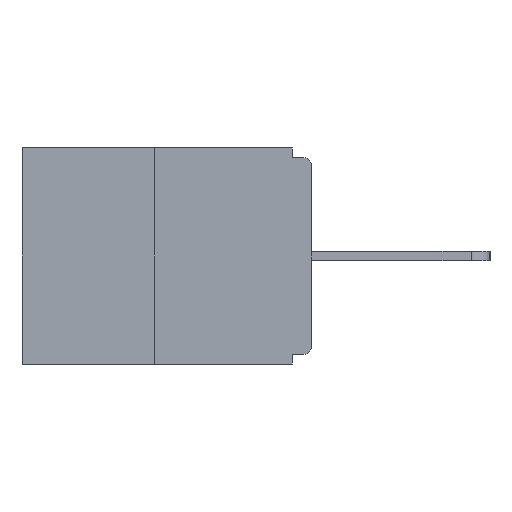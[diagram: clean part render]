
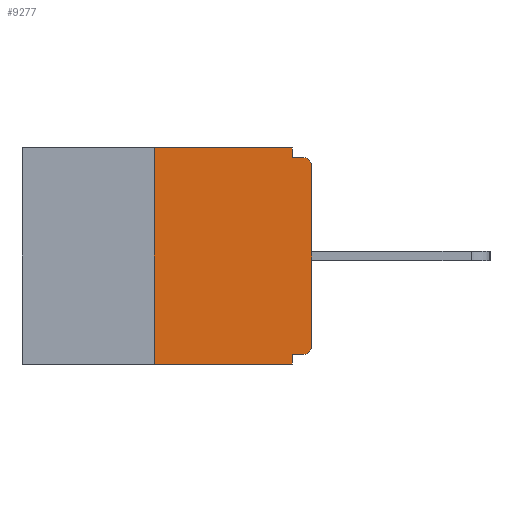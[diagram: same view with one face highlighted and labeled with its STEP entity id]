
A CAD part, left-side view. The second image highlights one B-rep face of the part: STEP entity #9277.
In plain terms, the highlighted planar face has unit normal (-1, 0, 0).
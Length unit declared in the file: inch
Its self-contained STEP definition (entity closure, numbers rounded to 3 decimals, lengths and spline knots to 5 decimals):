
#47 = CARTESIAN_POINT ( 'NONE',  ( 0., 0., -0.015 ) ) ;
#317 = DIRECTION ( 'NONE',  ( 0., 1., 0. ) ) ;
#396 = CARTESIAN_POINT ( 'NONE',  ( 0., 0.25, 0. ) ) ;
#550 = CIRCLE ( 'NONE', #8208, 0.015 ) ;
#909 = VERTEX_POINT ( 'NONE', #8559 ) ;
#1046 = DIRECTION ( 'NONE',  ( 0., 0., 1. ) ) ;
#1180 = VECTOR ( 'NONE', #14859, 39.37008 ) ;
#1407 = LINE ( 'NONE', #47, #1180 ) ;
#1647 = VECTOR ( 'NONE', #11227, 39.37008 ) ;
#1730 = CARTESIAN_POINT ( 'NONE',  ( 0., 0., -0.328 ) ) ;
#1750 = VECTOR ( 'NONE', #12781, 39.37008 ) ;
#1773 = DIRECTION ( 'NONE',  ( -1., 0., 0. ) ) ;
#2042 = EDGE_CURVE ( 'NONE', #14101, #11144, #2411, .T. ) ;
#2411 = LINE ( 'NONE', #2553, #12735 ) ;
#2553 = CARTESIAN_POINT ( 'NONE',  ( 0., 0., 0. ) ) ;
#2626 = ORIENTED_EDGE ( 'NONE', *, *, #10121, .F. ) ;
#2649 = CARTESIAN_POINT ( 'NONE',  ( 0., 0., -0.313 ) ) ;
#3064 = ORIENTED_EDGE ( 'NONE', *, *, #10946, .T. ) ;
#3123 = EDGE_LOOP ( 'NONE', ( #6985, #7214, #9758, #12051, #2626, #3064, #4207, #6616, #13733, #9381 ) ) ;
#3523 = DIRECTION ( 'NONE',  ( 0., 0., -1. ) ) ;
#3637 = LINE ( 'NONE', #9335, #1750 ) ;
#3724 = VECTOR ( 'NONE', #7939, 39.37008 ) ;
#3832 = CARTESIAN_POINT ( 'NONE',  ( 0., 0.25, -0.343 ) ) ;
#4206 = VERTEX_POINT ( 'NONE', #8380 ) ;
#4207 = ORIENTED_EDGE ( 'NONE', *, *, #2042, .T. ) ;
#4418 = VERTEX_POINT ( 'NONE', #11089 ) ;
#4456 = EDGE_CURVE ( 'NONE', #4206, #909, #5824, .T. ) ;
#5024 = VERTEX_POINT ( 'NONE', #8567 ) ;
#5153 = EDGE_CURVE ( 'NONE', #5024, #6578, #14577, .T. ) ;
#5521 = CARTESIAN_POINT ( 'NONE',  ( 0., 0., -0.03 ) ) ;
#5589 = DIRECTION ( 'NONE',  ( 0., 0., -1. ) ) ;
#5775 = FACE_OUTER_BOUND ( 'NONE', #3123, .T. ) ;
#5824 = LINE ( 'NONE', #10176, #3724 ) ;
#5860 = DIRECTION ( 'NONE',  ( 0., 0., 1. ) ) ;
#5984 = AXIS2_PLACEMENT_3D ( 'NONE', #9222, #13804, #3523 ) ;
#6578 = VERTEX_POINT ( 'NONE', #9167 ) ;
#6616 = ORIENTED_EDGE ( 'NONE', *, *, #7360, .T. ) ;
#6860 = AXIS2_PLACEMENT_3D ( 'NONE', #9583, #1773, #10788 ) ;
#6985 = ORIENTED_EDGE ( 'NONE', *, *, #7396, .F. ) ;
#7214 = ORIENTED_EDGE ( 'NONE', *, *, #12760, .F. ) ;
#7360 = EDGE_CURVE ( 'NONE', #11144, #4418, #550, .T. ) ;
#7396 = EDGE_CURVE ( 'NONE', #8554, #4206, #3637, .T. ) ;
#7939 = DIRECTION ( 'NONE',  ( 0., 0., -1. ) ) ;
#7997 = CARTESIAN_POINT ( 'NONE',  ( 0., 0.015, -0.03 ) ) ;
#8208 = AXIS2_PLACEMENT_3D ( 'NONE', #7997, #11525, #5589 ) ;
#8380 = CARTESIAN_POINT ( 'NONE',  ( 0., 0.031, 0. ) ) ;
#8554 = VERTEX_POINT ( 'NONE', #396 ) ;
#8559 = CARTESIAN_POINT ( 'NONE',  ( 0., 0.031, -0.015 ) ) ;
#8567 = CARTESIAN_POINT ( 'NONE',  ( 0., 0.031, -0.328 ) ) ;
#8672 = LINE ( 'NONE', #10094, #1647 ) ;
#9078 = CARTESIAN_POINT ( 'NONE',  ( 0., 0.25, 0. ) ) ;
#9167 = CARTESIAN_POINT ( 'NONE',  ( 0., 0.031, -0.343 ) ) ;
#9222 = CARTESIAN_POINT ( 'NONE',  ( 0., 0.46, 0. ) ) ;
#9254 = EDGE_CURVE ( 'NONE', #909, #4418, #1407, .T. ) ;
#9277 = ADVANCED_FACE ( 'NONE', ( #5775 ), #10344, .F. ) ;
#9335 = CARTESIAN_POINT ( 'NONE',  ( 0., 0.46, 0. ) ) ;
#9381 = ORIENTED_EDGE ( 'NONE', *, *, #4456, .F. ) ;
#9583 = CARTESIAN_POINT ( 'NONE',  ( 0., 0.015, -0.313 ) ) ;
#9758 = ORIENTED_EDGE ( 'NONE', *, *, #11175, .T. ) ;
#10094 = CARTESIAN_POINT ( 'NONE',  ( 0., 0.46, -0.343 ) ) ;
#10121 = EDGE_CURVE ( 'NONE', #14429, #5024, #11041, .T. ) ;
#10176 = CARTESIAN_POINT ( 'NONE',  ( 0., 0.031, 0. ) ) ;
#10344 = PLANE ( 'NONE',  #5984 ) ;
#10509 = VERTEX_POINT ( 'NONE', #3832 ) ;
#10788 = DIRECTION ( 'NONE',  ( 0., 0., -1. ) ) ;
#10946 = EDGE_CURVE ( 'NONE', #14429, #14101, #13099, .T. ) ;
#11041 = LINE ( 'NONE', #1730, #12155 ) ;
#11079 = VECTOR ( 'NONE', #12160, 39.37008 ) ;
#11089 = CARTESIAN_POINT ( 'NONE',  ( 0., 0.015, -0.015 ) ) ;
#11113 = CARTESIAN_POINT ( 'NONE',  ( 0., 0.031, -0.343 ) ) ;
#11144 = VERTEX_POINT ( 'NONE', #5521 ) ;
#11175 = EDGE_CURVE ( 'NONE', #10509, #6578, #8672, .T. ) ;
#11227 = DIRECTION ( 'NONE',  ( 0., -1., 0. ) ) ;
#11338 = LINE ( 'NONE', #9078, #11749 ) ;
#11525 = DIRECTION ( 'NONE',  ( -1., 0., 0. ) ) ;
#11749 = VECTOR ( 'NONE', #1046, 39.37008 ) ;
#12051 = ORIENTED_EDGE ( 'NONE', *, *, #5153, .F. ) ;
#12155 = VECTOR ( 'NONE', #317, 39.37008 ) ;
#12160 = DIRECTION ( 'NONE',  ( 0., 0., -1. ) ) ;
#12735 = VECTOR ( 'NONE', #5860, 39.37008 ) ;
#12760 = EDGE_CURVE ( 'NONE', #10509, #8554, #11338, .T. ) ;
#12781 = DIRECTION ( 'NONE',  ( 0., -1., 0. ) ) ;
#13099 = CIRCLE ( 'NONE', #6860, 0.015 ) ;
#13733 = ORIENTED_EDGE ( 'NONE', *, *, #9254, .F. ) ;
#13804 = DIRECTION ( 'NONE',  ( 1., 0., 0. ) ) ;
#13944 = CARTESIAN_POINT ( 'NONE',  ( 0., 0.015, -0.328 ) ) ;
#14101 = VERTEX_POINT ( 'NONE', #2649 ) ;
#14429 = VERTEX_POINT ( 'NONE', #13944 ) ;
#14577 = LINE ( 'NONE', #11113, #11079 ) ;
#14859 = DIRECTION ( 'NONE',  ( 0., -1., 0. ) ) ;
